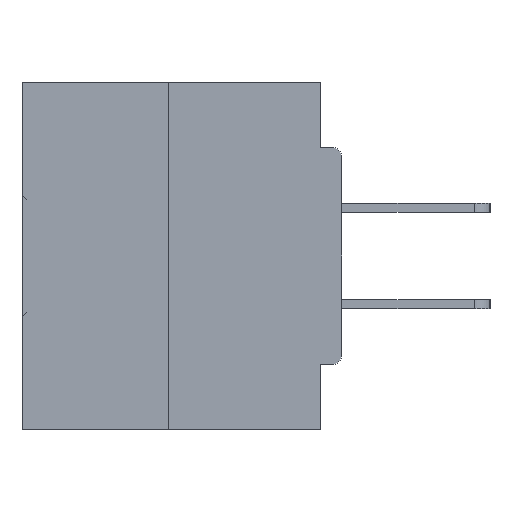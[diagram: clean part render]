
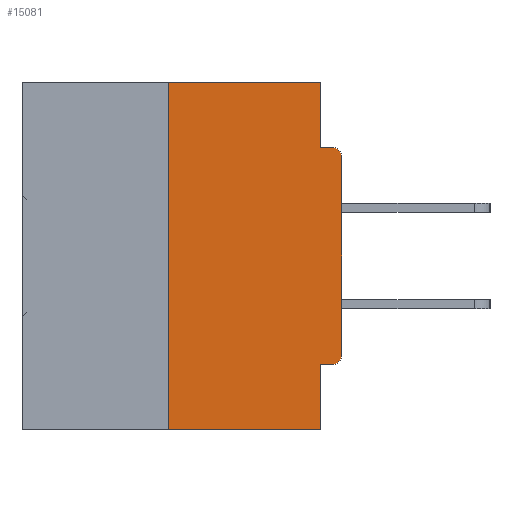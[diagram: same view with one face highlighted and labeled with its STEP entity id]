
A CAD part, left-side view. The second image highlights one B-rep face of the part: STEP entity #15081.
In plain terms, the highlighted planar face has unit normal (-1, 0, 0).
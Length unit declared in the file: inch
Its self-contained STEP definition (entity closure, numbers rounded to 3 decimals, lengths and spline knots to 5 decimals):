
#351 = EDGE_CURVE ( 'NONE', #28726, #43335, #43353, .T. ) ;
#692 = VERTEX_POINT ( 'NONE', #39374 ) ;
#2136 = CIRCLE ( 'NONE', #11008, 0.015 ) ;
#2243 = ORIENTED_EDGE ( 'NONE', *, *, #12475, .T. ) ;
#2435 = DIRECTION ( 'NONE',  ( 0., 0., 1. ) ) ;
#2559 = DIRECTION ( 'NONE',  ( 0., 0., -1. ) ) ;
#2561 = VECTOR ( 'NONE', #9410, 39.37008 ) ;
#3260 = VERTEX_POINT ( 'NONE', #13090 ) ;
#3297 = CARTESIAN_POINT ( 'NONE',  ( 0., 0., -0.3915 ) ) ;
#3654 = AXIS2_PLACEMENT_3D ( 'NONE', #19979, #24372, #2559 ) ;
#4764 = EDGE_CURVE ( 'NONE', #17643, #28726, #41589, .T. ) ;
#5346 = VECTOR ( 'NONE', #2435, 39.37008 ) ;
#5694 = VECTOR ( 'NONE', #25192, 39.37008 ) ;
#5862 = VECTOR ( 'NONE', #41170, 39.37008 ) ;
#6176 = LINE ( 'NONE', #9680, #22577 ) ;
#6333 = CARTESIAN_POINT ( 'NONE',  ( 0., 0.25, 0. ) ) ;
#8142 = CARTESIAN_POINT ( 'NONE',  ( 0., 0.25, -0.5 ) ) ;
#8989 = CARTESIAN_POINT ( 'NONE',  ( 0., 0., 0. ) ) ;
#9410 = DIRECTION ( 'NONE',  ( 0., 0., -1. ) ) ;
#9680 = CARTESIAN_POINT ( 'NONE',  ( 0., 0.46, -0.5 ) ) ;
#9844 = CARTESIAN_POINT ( 'NONE',  ( 0., 0.25, 0. ) ) ;
#11008 = AXIS2_PLACEMENT_3D ( 'NONE', #21208, #35122, #17751 ) ;
#11433 = ORIENTED_EDGE ( 'NONE', *, *, #31086, .T. ) ;
#11958 = CARTESIAN_POINT ( 'NONE',  ( 0., 0.031, -0.5 ) ) ;
#12475 = EDGE_CURVE ( 'NONE', #17643, #40010, #6176, .T. ) ;
#12609 = LINE ( 'NONE', #37171, #39572 ) ;
#12667 = CARTESIAN_POINT ( 'NONE',  ( 0., 0.031, 0. ) ) ;
#12695 = LINE ( 'NONE', #8989, #5862 ) ;
#13004 = FACE_OUTER_BOUND ( 'NONE', #44767, .T. ) ;
#13090 = CARTESIAN_POINT ( 'NONE',  ( 0., 0., -0.1085 ) ) ;
#13695 = ORIENTED_EDGE ( 'NONE', *, *, #24776, .T. ) ;
#14072 = AXIS2_PLACEMENT_3D ( 'NONE', #25903, #26109, #22635 ) ;
#14581 = ORIENTED_EDGE ( 'NONE', *, *, #33539, .F. ) ;
#15081 = ADVANCED_FACE ( 'NONE', ( #13004 ), #24132, .F. ) ;
#15565 = CARTESIAN_POINT ( 'NONE',  ( 0., 0.46, 0. ) ) ;
#15839 = DIRECTION ( 'NONE',  ( 0., -1., 0. ) ) ;
#17643 = VERTEX_POINT ( 'NONE', #8142 ) ;
#17751 = DIRECTION ( 'NONE',  ( 0., 0., -1. ) ) ;
#17931 = CARTESIAN_POINT ( 'NONE',  ( 0., 0.031, -0.5 ) ) ;
#18540 = EDGE_CURVE ( 'NONE', #43335, #692, #40689, .T. ) ;
#19979 = CARTESIAN_POINT ( 'NONE',  ( 0., 0.46, 0. ) ) ;
#20429 = ORIENTED_EDGE ( 'NONE', *, *, #18540, .F. ) ;
#21208 = CARTESIAN_POINT ( 'NONE',  ( 0., 0.015, -0.1085 ) ) ;
#21240 = LINE ( 'NONE', #11958, #5694 ) ;
#22577 = VECTOR ( 'NONE', #27757, 39.37008 ) ;
#22635 = DIRECTION ( 'NONE',  ( 0., 0., -1. ) ) ;
#22641 = EDGE_CURVE ( 'NONE', #27465, #29100, #29501, .T. ) ;
#23674 = CIRCLE ( 'NONE', #14072, 0.015 ) ;
#24132 = PLANE ( 'NONE',  #3654 ) ;
#24370 = CARTESIAN_POINT ( 'NONE',  ( 0., 0.015, -0.4065 ) ) ;
#24372 = DIRECTION ( 'NONE',  ( 1., 0., 0. ) ) ;
#24776 = EDGE_CURVE ( 'NONE', #27465, #35101, #23674, .T. ) ;
#25192 = DIRECTION ( 'NONE',  ( 0., 0., -1. ) ) ;
#25903 = CARTESIAN_POINT ( 'NONE',  ( 0., 0.015, -0.3915 ) ) ;
#26109 = DIRECTION ( 'NONE',  ( -1., 0., 0. ) ) ;
#27030 = EDGE_CURVE ( 'NONE', #29100, #40010, #21240, .T. ) ;
#27465 = VERTEX_POINT ( 'NONE', #24370 ) ;
#27757 = DIRECTION ( 'NONE',  ( 0., -1., 0. ) ) ;
#28726 = VERTEX_POINT ( 'NONE', #6333 ) ;
#29100 = VERTEX_POINT ( 'NONE', #40962 ) ;
#29469 = VERTEX_POINT ( 'NONE', #32182 ) ;
#29501 = LINE ( 'NONE', #29948, #31702 ) ;
#29596 = ORIENTED_EDGE ( 'NONE', *, *, #37044, .T. ) ;
#29948 = CARTESIAN_POINT ( 'NONE',  ( 0., 0., -0.4065 ) ) ;
#31086 = EDGE_CURVE ( 'NONE', #35101, #3260, #12695, .T. ) ;
#31702 = VECTOR ( 'NONE', #33225, 39.37008 ) ;
#32182 = CARTESIAN_POINT ( 'NONE',  ( 0., 0.015, -0.0935 ) ) ;
#32763 = ORIENTED_EDGE ( 'NONE', *, *, #22641, .F. ) ;
#33225 = DIRECTION ( 'NONE',  ( 0., 1., 0. ) ) ;
#33539 = EDGE_CURVE ( 'NONE', #692, #29469, #12609, .T. ) ;
#35101 = VERTEX_POINT ( 'NONE', #3297 ) ;
#35122 = DIRECTION ( 'NONE',  ( -1., 0., 0. ) ) ;
#37044 = EDGE_CURVE ( 'NONE', #3260, #29469, #2136, .T. ) ;
#37171 = CARTESIAN_POINT ( 'NONE',  ( 0., 0., -0.0935 ) ) ;
#37786 = ORIENTED_EDGE ( 'NONE', *, *, #27030, .F. ) ;
#39374 = CARTESIAN_POINT ( 'NONE',  ( 0., 0.031, -0.0935 ) ) ;
#39572 = VECTOR ( 'NONE', #15839, 39.37008 ) ;
#40010 = VERTEX_POINT ( 'NONE', #17931 ) ;
#40573 = DIRECTION ( 'NONE',  ( 0., -1., 0. ) ) ;
#40619 = ORIENTED_EDGE ( 'NONE', *, *, #4764, .F. ) ;
#40689 = LINE ( 'NONE', #12667, #2561 ) ;
#40901 = CARTESIAN_POINT ( 'NONE',  ( 0., 0.031, 0. ) ) ;
#40962 = CARTESIAN_POINT ( 'NONE',  ( 0., 0.031, -0.4065 ) ) ;
#41170 = DIRECTION ( 'NONE',  ( 0., 0., 1. ) ) ;
#41589 = LINE ( 'NONE', #9844, #5346 ) ;
#43025 = VECTOR ( 'NONE', #40573, 39.37008 ) ;
#43335 = VERTEX_POINT ( 'NONE', #40901 ) ;
#43353 = LINE ( 'NONE', #15565, #43025 ) ;
#44354 = ORIENTED_EDGE ( 'NONE', *, *, #351, .F. ) ;
#44767 = EDGE_LOOP ( 'NONE', ( #44354, #40619, #2243, #37786, #32763, #13695, #11433, #29596, #14581, #20429 ) ) ;
